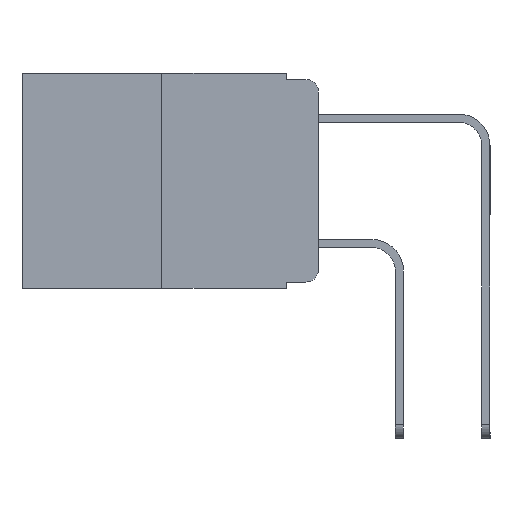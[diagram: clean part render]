
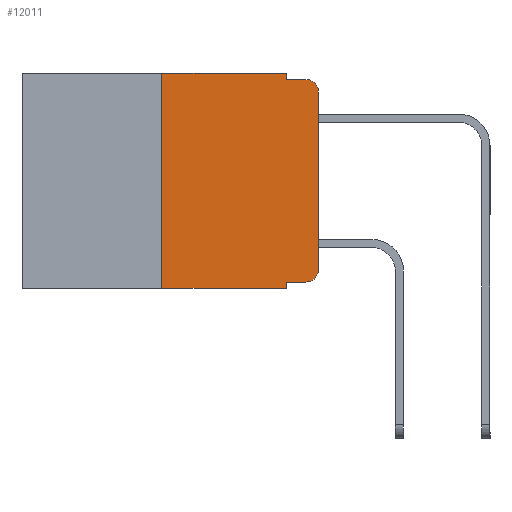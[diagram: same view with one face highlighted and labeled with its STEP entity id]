
A CAD part, left-side view. The second image highlights one B-rep face of the part: STEP entity #12011.
In plain terms, the highlighted planar face has unit normal (-1, 0, 0).
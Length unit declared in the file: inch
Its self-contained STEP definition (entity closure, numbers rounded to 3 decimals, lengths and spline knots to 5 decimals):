
#536 = VERTEX_POINT ( 'NONE', #26047 ) ;
#612 = DIRECTION ( 'NONE',  ( -1., 0., 0. ) ) ;
#1358 = DIRECTION ( 'NONE',  ( 0., -1., 0. ) ) ;
#1994 = ORIENTED_EDGE ( 'NONE', *, *, #19585, .T. ) ;
#2031 = DIRECTION ( 'NONE',  ( 0., -1., 0. ) ) ;
#2214 = DIRECTION ( 'NONE',  ( 0., -1., 0. ) ) ;
#2357 = ORIENTED_EDGE ( 'NONE', *, *, #23632, .T. ) ;
#2407 = VECTOR ( 'NONE', #2214, 39.37008 ) ;
#2826 = VECTOR ( 'NONE', #12383, 39.37008 ) ;
#3347 = CARTESIAN_POINT ( 'NONE',  ( 0., 0.25, 0. ) ) ;
#3375 = ORIENTED_EDGE ( 'NONE', *, *, #15538, .F. ) ;
#3830 = LINE ( 'NONE', #19869, #25796 ) ;
#4467 = VERTEX_POINT ( 'NONE', #12532 ) ;
#4829 = CARTESIAN_POINT ( 'NONE',  ( 0., 0.02, -0.313 ) ) ;
#5127 = CIRCLE ( 'NONE', #6531, 0.02 ) ;
#5445 = ORIENTED_EDGE ( 'NONE', *, *, #23543, .F. ) ;
#5582 = VECTOR ( 'NONE', #6661, 39.37008 ) ;
#6531 = AXIS2_PLACEMENT_3D ( 'NONE', #13331, #612, #15363 ) ;
#6661 = DIRECTION ( 'NONE',  ( 0., -1., 0. ) ) ;
#6787 = ORIENTED_EDGE ( 'NONE', *, *, #16793, .T. ) ;
#7008 = DIRECTION ( 'NONE',  ( 0., 0., -1. ) ) ;
#7572 = DIRECTION ( 'NONE',  ( 0., 0., 1. ) ) ;
#7738 = EDGE_CURVE ( 'NONE', #9612, #22036, #5127, .T. ) ;
#8094 = VECTOR ( 'NONE', #17494, 39.37008 ) ;
#8204 = CARTESIAN_POINT ( 'NONE',  ( 0., 0., -0.313 ) ) ;
#8314 = EDGE_LOOP ( 'NONE', ( #1994, #13285, #3375, #19967, #26645, #5445, #6787, #12322, #2357, #13618 ) ) ;
#8595 = VERTEX_POINT ( 'NONE', #8204 ) ;
#9268 = CARTESIAN_POINT ( 'NONE',  ( 0., 0.02, -0.01 ) ) ;
#9612 = VERTEX_POINT ( 'NONE', #11883 ) ;
#10689 = CIRCLE ( 'NONE', #18673, 0.02 ) ;
#11883 = CARTESIAN_POINT ( 'NONE',  ( 0., 0., -0.03 ) ) ;
#12011 = ADVANCED_FACE ( 'NONE', ( #20735 ), #20233, .F. ) ;
#12086 = EDGE_CURVE ( 'NONE', #4467, #24367, #19453, .T. ) ;
#12121 = DIRECTION ( 'NONE',  ( 1., 0., 0. ) ) ;
#12322 = ORIENTED_EDGE ( 'NONE', *, *, #17669, .F. ) ;
#12383 = DIRECTION ( 'NONE',  ( 0., 0., -1. ) ) ;
#12454 = LINE ( 'NONE', #16960, #5582 ) ;
#12532 = CARTESIAN_POINT ( 'NONE',  ( 0., 0.051, 0. ) ) ;
#12540 = VECTOR ( 'NONE', #15803, 39.37008 ) ;
#12698 = VERTEX_POINT ( 'NONE', #14417 ) ;
#12706 = CARTESIAN_POINT ( 'NONE',  ( 0., 0.473, 0. ) ) ;
#12751 = CARTESIAN_POINT ( 'NONE',  ( 0., 0.02, -0.333 ) ) ;
#12780 = CARTESIAN_POINT ( 'NONE',  ( 0., 0.473, -0.343 ) ) ;
#13178 = VERTEX_POINT ( 'NONE', #14027 ) ;
#13285 = ORIENTED_EDGE ( 'NONE', *, *, #7738, .T. ) ;
#13331 = CARTESIAN_POINT ( 'NONE',  ( 0., 0.02, -0.03 ) ) ;
#13618 = ORIENTED_EDGE ( 'NONE', *, *, #21968, .T. ) ;
#14027 = CARTESIAN_POINT ( 'NONE',  ( 0., 0.051, -0.343 ) ) ;
#14359 = CARTESIAN_POINT ( 'NONE',  ( 0., 0.051, -0.01 ) ) ;
#14417 = CARTESIAN_POINT ( 'NONE',  ( 0., 0.051, -0.333 ) ) ;
#15197 = VERTEX_POINT ( 'NONE', #3347 ) ;
#15363 = DIRECTION ( 'NONE',  ( 0., 0., -1. ) ) ;
#15538 = EDGE_CURVE ( 'NONE', #24367, #22036, #12454, .T. ) ;
#15803 = DIRECTION ( 'NONE',  ( 0., 0., 1. ) ) ;
#15929 = AXIS2_PLACEMENT_3D ( 'NONE', #24300, #12121, #26355 ) ;
#16036 = LINE ( 'NONE', #26216, #26235 ) ;
#16793 = EDGE_CURVE ( 'NONE', #536, #13178, #20359, .T. ) ;
#16960 = CARTESIAN_POINT ( 'NONE',  ( 0., 0.051, -0.01 ) ) ;
#17494 = DIRECTION ( 'NONE',  ( 0., 0., -1. ) ) ;
#17669 = EDGE_CURVE ( 'NONE', #12698, #13178, #23795, .T. ) ;
#18673 = AXIS2_PLACEMENT_3D ( 'NONE', #4829, #19327, #7008 ) ;
#19327 = DIRECTION ( 'NONE',  ( -1., 0., 0. ) ) ;
#19364 = VERTEX_POINT ( 'NONE', #12751 ) ;
#19453 = LINE ( 'NONE', #26529, #2826 ) ;
#19585 = EDGE_CURVE ( 'NONE', #8595, #9612, #3830, .T. ) ;
#19727 = CARTESIAN_POINT ( 'NONE',  ( 0., 0.25, 0. ) ) ;
#19869 = CARTESIAN_POINT ( 'NONE',  ( 0., 0., 0. ) ) ;
#19967 = ORIENTED_EDGE ( 'NONE', *, *, #12086, .F. ) ;
#20233 = PLANE ( 'NONE',  #15929 ) ;
#20359 = LINE ( 'NONE', #12780, #2407 ) ;
#20735 = FACE_OUTER_BOUND ( 'NONE', #8314, .T. ) ;
#21968 = EDGE_CURVE ( 'NONE', #19364, #8595, #10689, .T. ) ;
#22036 = VERTEX_POINT ( 'NONE', #9268 ) ;
#22463 = EDGE_CURVE ( 'NONE', #15197, #4467, #25666, .T. ) ;
#23376 = LINE ( 'NONE', #19727, #12540 ) ;
#23543 = EDGE_CURVE ( 'NONE', #536, #15197, #23376, .T. ) ;
#23596 = CARTESIAN_POINT ( 'NONE',  ( 0., 0.051, 0. ) ) ;
#23632 = EDGE_CURVE ( 'NONE', #12698, #19364, #16036, .T. ) ;
#23795 = LINE ( 'NONE', #23596, #8094 ) ;
#24300 = CARTESIAN_POINT ( 'NONE',  ( 0., 0.473, 0. ) ) ;
#24367 = VERTEX_POINT ( 'NONE', #14359 ) ;
#25031 = VECTOR ( 'NONE', #2031, 39.37008 ) ;
#25666 = LINE ( 'NONE', #12706, #25031 ) ;
#25796 = VECTOR ( 'NONE', #7572, 39.37008 ) ;
#26047 = CARTESIAN_POINT ( 'NONE',  ( 0., 0.25, -0.343 ) ) ;
#26216 = CARTESIAN_POINT ( 'NONE',  ( 0., 0.051, -0.333 ) ) ;
#26235 = VECTOR ( 'NONE', #1358, 39.37008 ) ;
#26355 = DIRECTION ( 'NONE',  ( 0., 0., -1. ) ) ;
#26529 = CARTESIAN_POINT ( 'NONE',  ( 0., 0.051, 0. ) ) ;
#26645 = ORIENTED_EDGE ( 'NONE', *, *, #22463, .F. ) ;
